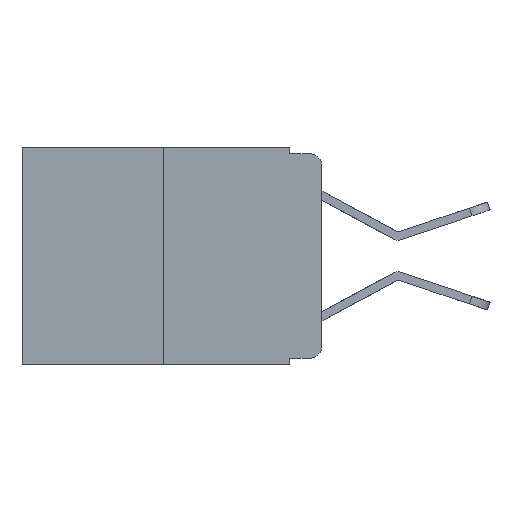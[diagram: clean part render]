
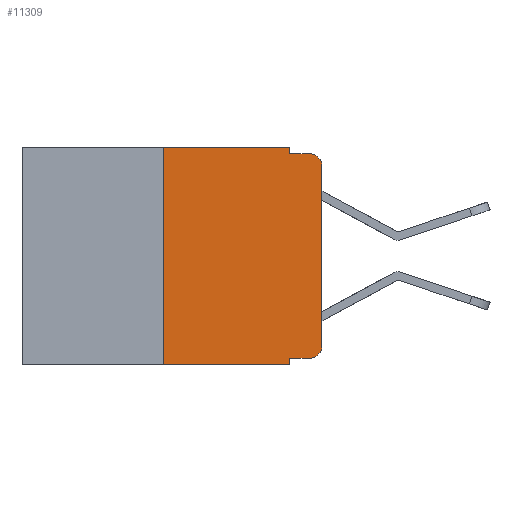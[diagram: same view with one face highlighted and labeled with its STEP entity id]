
A CAD part, left-side view. The second image highlights one B-rep face of the part: STEP entity #11309.
In plain terms, the highlighted planar face has unit normal (-1, 0, 0).
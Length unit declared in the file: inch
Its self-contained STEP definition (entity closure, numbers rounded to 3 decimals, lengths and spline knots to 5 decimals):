
#23 = DIRECTION ( 'NONE',  ( 0., 0., -1. ) ) ;
#59 = CARTESIAN_POINT ( 'NONE',  ( 0., 0., -0.03 ) ) ;
#746 = CARTESIAN_POINT ( 'NONE',  ( 0., 0., 0. ) ) ;
#877 = VECTOR ( 'NONE', #14268, 39.37008 ) ;
#983 = VERTEX_POINT ( 'NONE', #3703 ) ;
#1317 = EDGE_CURVE ( 'NONE', #8063, #5107, #6562, .T. ) ;
#1379 = EDGE_CURVE ( 'NONE', #8976, #7708, #12992, .T. ) ;
#1715 = FACE_OUTER_BOUND ( 'NONE', #16649, .T. ) ;
#1750 = CARTESIAN_POINT ( 'NONE',  ( 0., 0.25, 0. ) ) ;
#1958 = AXIS2_PLACEMENT_3D ( 'NONE', #2429, #11663, #3750 ) ;
#2118 = LINE ( 'NONE', #3982, #8744 ) ;
#2138 = ORIENTED_EDGE ( 'NONE', *, *, #7966, .F. ) ;
#2249 = DIRECTION ( 'NONE',  ( 1., 0., 0. ) ) ;
#2283 = ORIENTED_EDGE ( 'NONE', *, *, #13717, .F. ) ;
#2321 = ORIENTED_EDGE ( 'NONE', *, *, #11361, .T. ) ;
#2428 = AXIS2_PLACEMENT_3D ( 'NONE', #13458, #5540, #14813 ) ;
#2429 = CARTESIAN_POINT ( 'NONE',  ( 0., 0.02, -0.313 ) ) ;
#2555 = DIRECTION ( 'NONE',  ( 0., -1., 0. ) ) ;
#2585 = VERTEX_POINT ( 'NONE', #59 ) ;
#2663 = EDGE_CURVE ( 'NONE', #2585, #14796, #16757, .T. ) ;
#2884 = CARTESIAN_POINT ( 'NONE',  ( 0., 0.25, -0.343 ) ) ;
#3115 = CARTESIAN_POINT ( 'NONE',  ( 0., 0.051, 0. ) ) ;
#3212 = ORIENTED_EDGE ( 'NONE', *, *, #1317, .F. ) ;
#3300 = VECTOR ( 'NONE', #2555, 39.37008 ) ;
#3415 = VERTEX_POINT ( 'NONE', #13027 ) ;
#3703 = CARTESIAN_POINT ( 'NONE',  ( 0., 0.051, -0.333 ) ) ;
#3750 = DIRECTION ( 'NONE',  ( 0., 0., -1. ) ) ;
#3982 = CARTESIAN_POINT ( 'NONE',  ( 0., 0.051, 0. ) ) ;
#4400 = ORIENTED_EDGE ( 'NONE', *, *, #6244, .T. ) ;
#4452 = CARTESIAN_POINT ( 'NONE',  ( 0., 0.051, -0.333 ) ) ;
#5107 = VERTEX_POINT ( 'NONE', #1750 ) ;
#5197 = VERTEX_POINT ( 'NONE', #5938 ) ;
#5337 = DIRECTION ( 'NONE',  ( 0., 0., -1. ) ) ;
#5540 = DIRECTION ( 'NONE',  ( -1., 0., 0. ) ) ;
#5759 = CARTESIAN_POINT ( 'NONE',  ( 0., 0.051, -0.01 ) ) ;
#5775 = EDGE_CURVE ( 'NONE', #7708, #2585, #10862, .T. ) ;
#5808 = ORIENTED_EDGE ( 'NONE', *, *, #2663, .T. ) ;
#5938 = CARTESIAN_POINT ( 'NONE',  ( 0., 0.051, -0.01 ) ) ;
#5998 = ORIENTED_EDGE ( 'NONE', *, *, #1379, .T. ) ;
#6032 = DIRECTION ( 'NONE',  ( 0., 0., 1. ) ) ;
#6200 = LINE ( 'NONE', #5759, #15961 ) ;
#6201 = CARTESIAN_POINT ( 'NONE',  ( 0., 0.473, 0. ) ) ;
#6205 = AXIS2_PLACEMENT_3D ( 'NONE', #6201, #2249, #11491 ) ;
#6244 = EDGE_CURVE ( 'NONE', #983, #8976, #12703, .T. ) ;
#6253 = DIRECTION ( 'NONE',  ( 0., 0., 1. ) ) ;
#6419 = LINE ( 'NONE', #10476, #3300 ) ;
#6489 = ORIENTED_EDGE ( 'NONE', *, *, #12741, .F. ) ;
#6562 = LINE ( 'NONE', #7590, #9879 ) ;
#7076 = DIRECTION ( 'NONE',  ( 0., -1., 0. ) ) ;
#7533 = VERTEX_POINT ( 'NONE', #3115 ) ;
#7590 = CARTESIAN_POINT ( 'NONE',  ( 0., 0.25, 0. ) ) ;
#7708 = VERTEX_POINT ( 'NONE', #11371 ) ;
#7934 = LINE ( 'NONE', #8902, #877 ) ;
#7966 = EDGE_CURVE ( 'NONE', #7533, #5197, #2118, .T. ) ;
#8063 = VERTEX_POINT ( 'NONE', #2884 ) ;
#8068 = ORIENTED_EDGE ( 'NONE', *, *, #5775, .T. ) ;
#8113 = ORIENTED_EDGE ( 'NONE', *, *, #13468, .F. ) ;
#8744 = VECTOR ( 'NONE', #5337, 39.37008 ) ;
#8902 = CARTESIAN_POINT ( 'NONE',  ( 0., 0.473, -0.343 ) ) ;
#8976 = VERTEX_POINT ( 'NONE', #11838 ) ;
#9209 = CARTESIAN_POINT ( 'NONE',  ( 0., 0.02, -0.01 ) ) ;
#9295 = CARTESIAN_POINT ( 'NONE',  ( 0., 0.051, 0. ) ) ;
#9725 = VECTOR ( 'NONE', #23, 39.37008 ) ;
#9879 = VECTOR ( 'NONE', #6253, 39.37008 ) ;
#10160 = PLANE ( 'NONE',  #6205 ) ;
#10476 = CARTESIAN_POINT ( 'NONE',  ( 0., 0.473, 0. ) ) ;
#10862 = LINE ( 'NONE', #746, #13996 ) ;
#11309 = ADVANCED_FACE ( 'NONE', ( #1715 ), #10160, .F. ) ;
#11361 = EDGE_CURVE ( 'NONE', #8063, #3415, #7934, .T. ) ;
#11371 = CARTESIAN_POINT ( 'NONE',  ( 0., 0., -0.313 ) ) ;
#11491 = DIRECTION ( 'NONE',  ( 0., 0., -1. ) ) ;
#11663 = DIRECTION ( 'NONE',  ( -1., 0., 0. ) ) ;
#11838 = CARTESIAN_POINT ( 'NONE',  ( 0., 0.02, -0.333 ) ) ;
#12703 = LINE ( 'NONE', #4452, #13129 ) ;
#12741 = EDGE_CURVE ( 'NONE', #983, #3415, #13255, .T. ) ;
#12992 = CIRCLE ( 'NONE', #1958, 0.02 ) ;
#13027 = CARTESIAN_POINT ( 'NONE',  ( 0., 0.051, -0.343 ) ) ;
#13129 = VECTOR ( 'NONE', #13696, 39.37008 ) ;
#13255 = LINE ( 'NONE', #9295, #9725 ) ;
#13458 = CARTESIAN_POINT ( 'NONE',  ( 0., 0.02, -0.03 ) ) ;
#13468 = EDGE_CURVE ( 'NONE', #5107, #7533, #6419, .T. ) ;
#13696 = DIRECTION ( 'NONE',  ( 0., -1., 0. ) ) ;
#13717 = EDGE_CURVE ( 'NONE', #5197, #14796, #6200, .T. ) ;
#13996 = VECTOR ( 'NONE', #6032, 39.37008 ) ;
#14268 = DIRECTION ( 'NONE',  ( 0., -1., 0. ) ) ;
#14796 = VERTEX_POINT ( 'NONE', #9209 ) ;
#14813 = DIRECTION ( 'NONE',  ( 0., 0., -1. ) ) ;
#15961 = VECTOR ( 'NONE', #7076, 39.37008 ) ;
#16649 = EDGE_LOOP ( 'NONE', ( #8068, #5808, #2283, #2138, #8113, #3212, #2321, #6489, #4400, #5998 ) ) ;
#16757 = CIRCLE ( 'NONE', #2428, 0.02 ) ;
